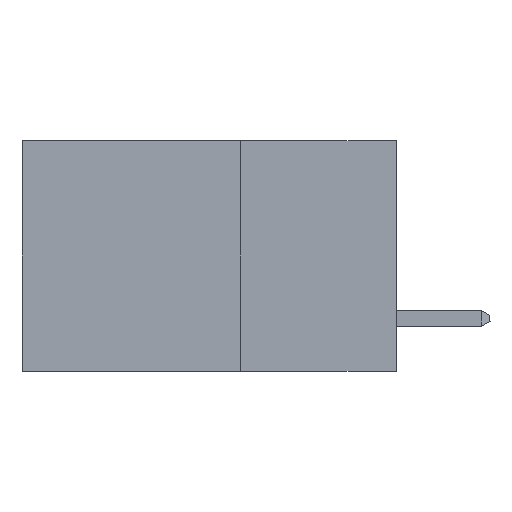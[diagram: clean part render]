
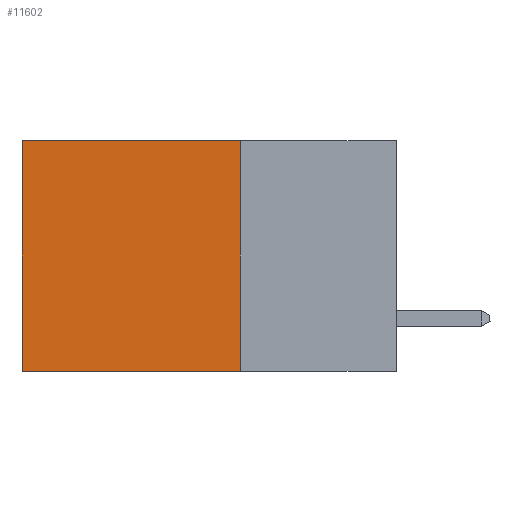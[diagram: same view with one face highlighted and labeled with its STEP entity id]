
A CAD part, left-side view. The second image highlights one B-rep face of the part: STEP entity #11602.
In plain terms, the highlighted planar face has unit normal (-1, 0, 0).
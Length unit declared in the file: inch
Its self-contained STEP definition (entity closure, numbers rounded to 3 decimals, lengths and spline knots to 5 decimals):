
#456 = ORIENTED_EDGE ( 'NONE', *, *, #11266, .F. ) ;
#811 = DIRECTION ( 'NONE',  ( 0., 0., -1. ) ) ;
#914 = EDGE_CURVE ( 'NONE', #3997, #2815, #4482, .T. ) ;
#1245 = DIRECTION ( 'NONE',  ( 0., 1., 0. ) ) ;
#1975 = DIRECTION ( 'NONE',  ( 0., 0., -1. ) ) ;
#2224 = VECTOR ( 'NONE', #9922, 39.37008 ) ;
#2491 = VECTOR ( 'NONE', #1245, 39.37008 ) ;
#2815 = VERTEX_POINT ( 'NONE', #11680 ) ;
#3090 = AXIS2_PLACEMENT_3D ( 'NONE', #4093, #7478, #811 ) ;
#3997 = VERTEX_POINT ( 'NONE', #8317 ) ;
#4093 = CARTESIAN_POINT ( 'NONE',  ( 0.298, 0.25, 0. ) ) ;
#4482 = LINE ( 'NONE', #9932, #2224 ) ;
#5119 = FACE_OUTER_BOUND ( 'NONE', #6315, .T. ) ;
#5368 = CARTESIAN_POINT ( 'NONE',  ( 0.298, 0.6, 0. ) ) ;
#6315 = EDGE_LOOP ( 'NONE', ( #10235, #456, #6904, #13083 ) ) ;
#6364 = PLANE ( 'NONE',  #3090 ) ;
#6904 = ORIENTED_EDGE ( 'NONE', *, *, #11014, .F. ) ;
#7046 = VECTOR ( 'NONE', #9698, 39.37008 ) ;
#7425 = CARTESIAN_POINT ( 'NONE',  ( 0.298, 0.25, -0.37 ) ) ;
#7478 = DIRECTION ( 'NONE',  ( 1., 0., 0. ) ) ;
#7531 = CARTESIAN_POINT ( 'NONE',  ( 0.298, 0.25, 0. ) ) ;
#8317 = CARTESIAN_POINT ( 'NONE',  ( 0.298, 0.25, 0. ) ) ;
#8901 = VERTEX_POINT ( 'NONE', #7425 ) ;
#8963 = CARTESIAN_POINT ( 'NONE',  ( 0.298, 0.25, -0.37 ) ) ;
#9698 = DIRECTION ( 'NONE',  ( 0., 0., -1. ) ) ;
#9862 = LINE ( 'NONE', #5368, #7046 ) ;
#9877 = LINE ( 'NONE', #8963, #2491 ) ;
#9922 = DIRECTION ( 'NONE',  ( 0., 1., 0. ) ) ;
#9932 = CARTESIAN_POINT ( 'NONE',  ( 0.298, 0.25, 0. ) ) ;
#10060 = VECTOR ( 'NONE', #1975, 39.37008 ) ;
#10234 = CARTESIAN_POINT ( 'NONE',  ( 0.298, 0.6, -0.37 ) ) ;
#10235 = ORIENTED_EDGE ( 'NONE', *, *, #11657, .T. ) ;
#10717 = LINE ( 'NONE', #7531, #10060 ) ;
#11014 = EDGE_CURVE ( 'NONE', #3997, #8901, #10717, .T. ) ;
#11266 = EDGE_CURVE ( 'NONE', #8901, #12711, #9877, .T. ) ;
#11602 = ADVANCED_FACE ( 'NONE', ( #5119 ), #6364, .F. ) ;
#11657 = EDGE_CURVE ( 'NONE', #2815, #12711, #9862, .T. ) ;
#11680 = CARTESIAN_POINT ( 'NONE',  ( 0.298, 0.6, 0. ) ) ;
#12711 = VERTEX_POINT ( 'NONE', #10234 ) ;
#13083 = ORIENTED_EDGE ( 'NONE', *, *, #914, .T. ) ;
